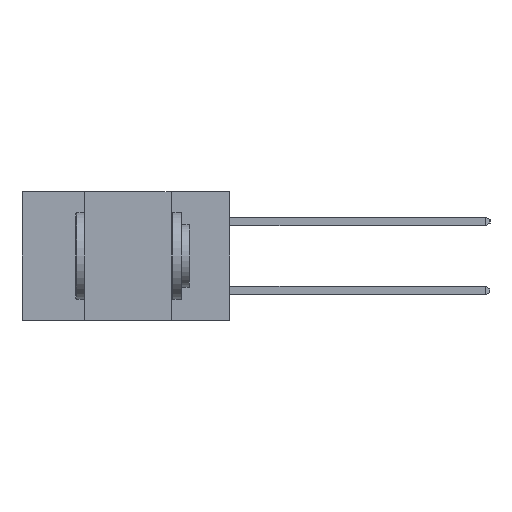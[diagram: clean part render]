
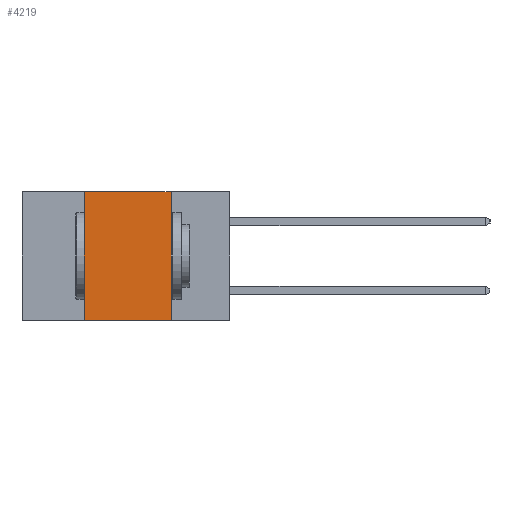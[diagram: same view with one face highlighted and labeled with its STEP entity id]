
A CAD part, left-side view. The second image highlights one B-rep face of the part: STEP entity #4219.
In plain terms, the highlighted planar face has unit normal (-1, 0, 0).
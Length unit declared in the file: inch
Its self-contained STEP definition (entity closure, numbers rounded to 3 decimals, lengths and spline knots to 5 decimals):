
#2057 = DIRECTION ( 'NONE',  ( 0., -1., 0. ) ) ;
#2223 = VECTOR ( 'NONE', #6224, 39.37008 ) ;
#2601 = VECTOR ( 'NONE', #15908, 39.37008 ) ;
#3193 = CARTESIAN_POINT ( 'NONE',  ( 0., 0.17, -0.37 ) ) ;
#3402 = ORIENTED_EDGE ( 'NONE', *, *, #15733, .F. ) ;
#3743 = EDGE_CURVE ( 'NONE', #17116, #5598, #4834, .T. ) ;
#4219 = ADVANCED_FACE ( 'NONE', ( #12194 ), #15923, .F. ) ;
#4291 = EDGE_LOOP ( 'NONE', ( #3402, #4773, #10094, #8503 ) ) ;
#4773 = ORIENTED_EDGE ( 'NONE', *, *, #7836, .F. ) ;
#4834 = LINE ( 'NONE', #18153, #8325 ) ;
#4977 = VERTEX_POINT ( 'NONE', #3193 ) ;
#5590 = CARTESIAN_POINT ( 'NONE',  ( 0., 0.6, -0.37 ) ) ;
#5598 = VERTEX_POINT ( 'NONE', #10988 ) ;
#5629 = DIRECTION ( 'NONE',  ( 0., 0., 1. ) ) ;
#6117 = CARTESIAN_POINT ( 'NONE',  ( 0., 0.6, 0. ) ) ;
#6169 = LINE ( 'NONE', #15029, #2223 ) ;
#6224 = DIRECTION ( 'NONE',  ( 0., 0., -1. ) ) ;
#7836 = EDGE_CURVE ( 'NONE', #5598, #8592, #11267, .T. ) ;
#8325 = VECTOR ( 'NONE', #5629, 39.37008 ) ;
#8388 = AXIS2_PLACEMENT_3D ( 'NONE', #6117, #15859, #15788 ) ;
#8503 = ORIENTED_EDGE ( 'NONE', *, *, #17349, .T. ) ;
#8592 = VERTEX_POINT ( 'NONE', #10486 ) ;
#9993 = LINE ( 'NONE', #5590, #2601 ) ;
#10094 = ORIENTED_EDGE ( 'NONE', *, *, #3743, .F. ) ;
#10486 = CARTESIAN_POINT ( 'NONE',  ( 0., 0.17, 0. ) ) ;
#10988 = CARTESIAN_POINT ( 'NONE',  ( 0., 0.42, 0. ) ) ;
#11190 = CARTESIAN_POINT ( 'NONE',  ( 0., 0.6, 0. ) ) ;
#11267 = LINE ( 'NONE', #11190, #18599 ) ;
#12194 = FACE_OUTER_BOUND ( 'NONE', #4291, .T. ) ;
#15029 = CARTESIAN_POINT ( 'NONE',  ( 0., 0.17, 0. ) ) ;
#15733 = EDGE_CURVE ( 'NONE', #8592, #4977, #6169, .T. ) ;
#15788 = DIRECTION ( 'NONE',  ( 0., 0., -1. ) ) ;
#15859 = DIRECTION ( 'NONE',  ( 1., 0., 0. ) ) ;
#15908 = DIRECTION ( 'NONE',  ( 0., -1., 0. ) ) ;
#15923 = PLANE ( 'NONE',  #8388 ) ;
#17116 = VERTEX_POINT ( 'NONE', #18224 ) ;
#17349 = EDGE_CURVE ( 'NONE', #17116, #4977, #9993, .T. ) ;
#18153 = CARTESIAN_POINT ( 'NONE',  ( 0., 0.42, 0. ) ) ;
#18224 = CARTESIAN_POINT ( 'NONE',  ( 0., 0.42, -0.37 ) ) ;
#18599 = VECTOR ( 'NONE', #2057, 39.37008 ) ;
